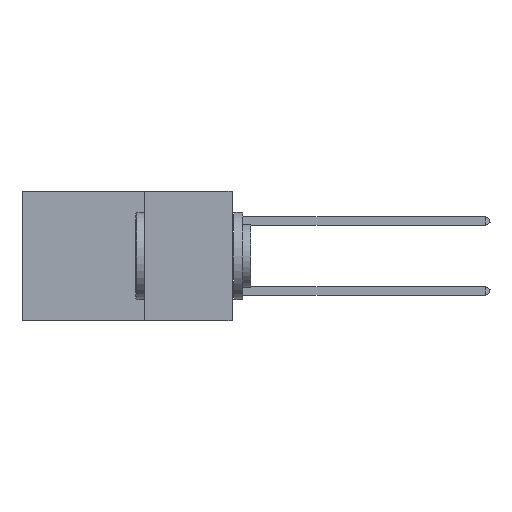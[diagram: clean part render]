
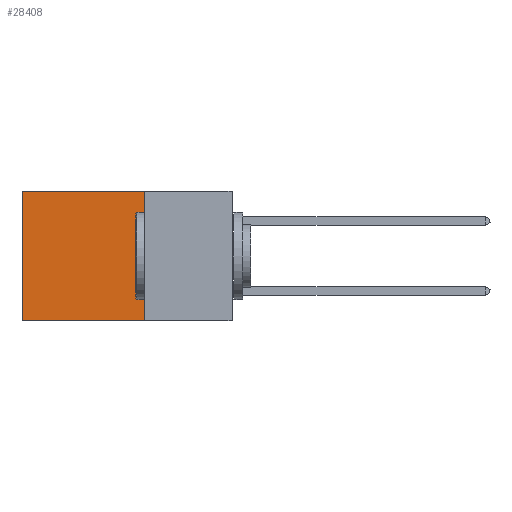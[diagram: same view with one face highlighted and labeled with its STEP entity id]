
A CAD part, left-side view. The second image highlights one B-rep face of the part: STEP entity #28408.
In plain terms, the highlighted planar face has unit normal (-1, 0, 0).
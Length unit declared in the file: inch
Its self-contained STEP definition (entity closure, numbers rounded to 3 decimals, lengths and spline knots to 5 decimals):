
#684 = AXIS2_PLACEMENT_3D ( 'NONE', #36458, #26979, #8239 ) ;
#943 = LINE ( 'NONE', #24170, #9200 ) ;
#2934 = LINE ( 'NONE', #27777, #36964 ) ;
#3833 = LINE ( 'NONE', #8163, #24912 ) ;
#4541 = EDGE_CURVE ( 'NONE', #5356, #10545, #3833, .T. ) ;
#5356 = VERTEX_POINT ( 'NONE', #27184 ) ;
#5616 = ORIENTED_EDGE ( 'NONE', *, *, #36348, .T. ) ;
#8163 = CARTESIAN_POINT ( 'NONE',  ( 0.2875, 0.25, 0. ) ) ;
#8239 = DIRECTION ( 'NONE',  ( 0., 0., -1. ) ) ;
#8879 = DIRECTION ( 'NONE',  ( 0., 1., 0. ) ) ;
#9200 = VECTOR ( 'NONE', #14610, 39.37008 ) ;
#9632 = CARTESIAN_POINT ( 'NONE',  ( 0.2875, 0.6, -0.37 ) ) ;
#10545 = VERTEX_POINT ( 'NONE', #29604 ) ;
#14407 = ORIENTED_EDGE ( 'NONE', *, *, #4541, .T. ) ;
#14610 = DIRECTION ( 'NONE',  ( 0., 0., -1. ) ) ;
#14868 = CARTESIAN_POINT ( 'NONE',  ( 0.2875, 0.25, -0.37 ) ) ;
#15290 = VECTOR ( 'NONE', #18683, 39.37008 ) ;
#17769 = LINE ( 'NONE', #27849, #15290 ) ;
#18683 = DIRECTION ( 'NONE',  ( 0., 1., 0. ) ) ;
#19280 = EDGE_CURVE ( 'NONE', #21940, #38605, #17769, .T. ) ;
#21178 = EDGE_LOOP ( 'NONE', ( #5616, #22721, #30337, #14407 ) ) ;
#21940 = VERTEX_POINT ( 'NONE', #14868 ) ;
#22721 = ORIENTED_EDGE ( 'NONE', *, *, #19280, .F. ) ;
#23160 = EDGE_CURVE ( 'NONE', #5356, #21940, #2934, .T. ) ;
#24170 = CARTESIAN_POINT ( 'NONE',  ( 0.2875, 0.6, 0. ) ) ;
#24912 = VECTOR ( 'NONE', #8879, 39.37008 ) ;
#26979 = DIRECTION ( 'NONE',  ( 1., 0., 0. ) ) ;
#27184 = CARTESIAN_POINT ( 'NONE',  ( 0.2875, 0.25, 0. ) ) ;
#27777 = CARTESIAN_POINT ( 'NONE',  ( 0.2875, 0.25, 0. ) ) ;
#27849 = CARTESIAN_POINT ( 'NONE',  ( 0.2875, 0.25, -0.37 ) ) ;
#28408 = ADVANCED_FACE ( 'NONE', ( #36340 ), #29762, .F. ) ;
#29604 = CARTESIAN_POINT ( 'NONE',  ( 0.2875, 0.6, 0. ) ) ;
#29762 = PLANE ( 'NONE',  #684 ) ;
#30337 = ORIENTED_EDGE ( 'NONE', *, *, #23160, .F. ) ;
#36340 = FACE_OUTER_BOUND ( 'NONE', #21178, .T. ) ;
#36348 = EDGE_CURVE ( 'NONE', #10545, #38605, #943, .T. ) ;
#36458 = CARTESIAN_POINT ( 'NONE',  ( 0.2875, 0.25, 0. ) ) ;
#36964 = VECTOR ( 'NONE', #40567, 39.37008 ) ;
#38605 = VERTEX_POINT ( 'NONE', #9632 ) ;
#40567 = DIRECTION ( 'NONE',  ( 0., 0., -1. ) ) ;
